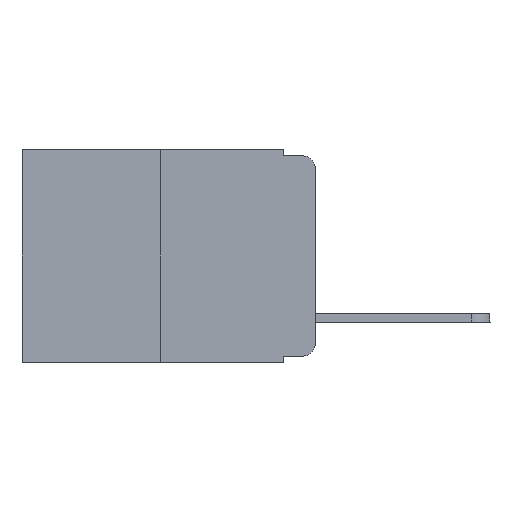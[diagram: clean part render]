
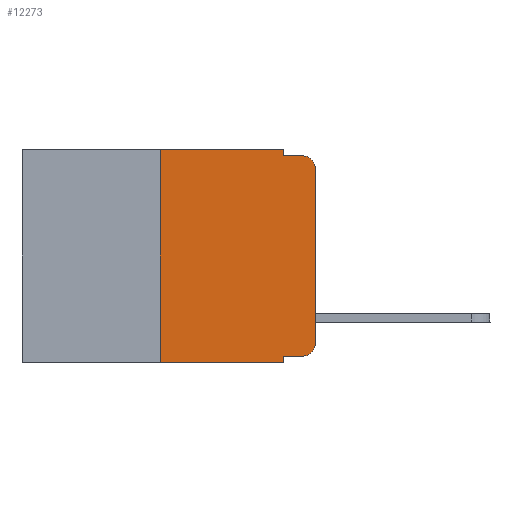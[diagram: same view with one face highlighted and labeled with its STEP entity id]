
A CAD part, left-side view. The second image highlights one B-rep face of the part: STEP entity #12273.
In plain terms, the highlighted planar face has unit normal (-1, 0, 0).
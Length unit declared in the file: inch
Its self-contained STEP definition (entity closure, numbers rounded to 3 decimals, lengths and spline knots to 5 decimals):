
#393 = VERTEX_POINT ( 'NONE', #15303 ) ;
#669 = EDGE_CURVE ( 'NONE', #393, #12281, #3960, .T. ) ;
#1210 = EDGE_CURVE ( 'NONE', #20038, #2780, #21327, .T. ) ;
#1405 = VERTEX_POINT ( 'NONE', #14627 ) ;
#1420 = EDGE_CURVE ( 'NONE', #5129, #18535, #2985, .T. ) ;
#2106 = FACE_OUTER_BOUND ( 'NONE', #10210, .T. ) ;
#2491 = LINE ( 'NONE', #22043, #21456 ) ;
#2536 = EDGE_CURVE ( 'NONE', #1405, #393, #21554, .T. ) ;
#2780 = VERTEX_POINT ( 'NONE', #20606 ) ;
#2985 = LINE ( 'NONE', #23862, #22255 ) ;
#3239 = EDGE_CURVE ( 'NONE', #6194, #11858, #14249, .T. ) ;
#3647 = CARTESIAN_POINT ( 'NONE',  ( 0., 0.02, -0.03 ) ) ;
#3960 = LINE ( 'NONE', #18649, #12678 ) ;
#5054 = ORIENTED_EDGE ( 'NONE', *, *, #14826, .F. ) ;
#5129 = VERTEX_POINT ( 'NONE', #21766 ) ;
#5661 = VECTOR ( 'NONE', #9989, 39.37008 ) ;
#5997 = DIRECTION ( 'NONE',  ( 0., -1., 0. ) ) ;
#6194 = VERTEX_POINT ( 'NONE', #10432 ) ;
#6291 = EDGE_CURVE ( 'NONE', #18881, #18535, #23233, .T. ) ;
#6604 = CARTESIAN_POINT ( 'NONE',  ( 0., 0.25, 0. ) ) ;
#6665 = DIRECTION ( 'NONE',  ( 1., 0., 0. ) ) ;
#6830 = ORIENTED_EDGE ( 'NONE', *, *, #1420, .F. ) ;
#7027 = EDGE_CURVE ( 'NONE', #11858, #20038, #16134, .T. ) ;
#8512 = CARTESIAN_POINT ( 'NONE',  ( 0., 0.051, -0.01 ) ) ;
#8839 = DIRECTION ( 'NONE',  ( 0., 0., -1. ) ) ;
#9484 = ORIENTED_EDGE ( 'NONE', *, *, #10793, .F. ) ;
#9567 = CARTESIAN_POINT ( 'NONE',  ( 0., 0., 0. ) ) ;
#9631 = VECTOR ( 'NONE', #12845, 39.37008 ) ;
#9811 = CARTESIAN_POINT ( 'NONE',  ( 0., 0.051, -0.333 ) ) ;
#9989 = DIRECTION ( 'NONE',  ( 0., -1., 0. ) ) ;
#10210 = EDGE_LOOP ( 'NONE', ( #11267, #16380, #9484, #14131, #15472, #5054, #15921, #6830, #18730, #19516 ) ) ;
#10270 = CARTESIAN_POINT ( 'NONE',  ( 0., 0.473, -0.343 ) ) ;
#10308 = DIRECTION ( 'NONE',  ( -1., 0., 0. ) ) ;
#10432 = CARTESIAN_POINT ( 'NONE',  ( 0., 0.02, -0.333 ) ) ;
#10793 = EDGE_CURVE ( 'NONE', #12281, #2780, #2491, .T. ) ;
#11267 = ORIENTED_EDGE ( 'NONE', *, *, #7027, .T. ) ;
#11858 = VERTEX_POINT ( 'NONE', #16925 ) ;
#12273 = ADVANCED_FACE ( 'NONE', ( #2106 ), #24027, .F. ) ;
#12281 = VERTEX_POINT ( 'NONE', #8512 ) ;
#12386 = DIRECTION ( 'NONE',  ( 0., 0., 1. ) ) ;
#12678 = VECTOR ( 'NONE', #20623, 39.37008 ) ;
#12823 = CARTESIAN_POINT ( 'NONE',  ( 0., 0.051, -0.343 ) ) ;
#12845 = DIRECTION ( 'NONE',  ( 0., -1., 0. ) ) ;
#13366 = CARTESIAN_POINT ( 'NONE',  ( 0., 0., -0.03 ) ) ;
#14131 = ORIENTED_EDGE ( 'NONE', *, *, #669, .F. ) ;
#14249 = CIRCLE ( 'NONE', #18062, 0.02 ) ;
#14353 = DIRECTION ( 'NONE',  ( 0., 0., -1. ) ) ;
#14627 = CARTESIAN_POINT ( 'NONE',  ( 0., 0.25, 0. ) ) ;
#14826 = EDGE_CURVE ( 'NONE', #18881, #1405, #17659, .T. ) ;
#15303 = CARTESIAN_POINT ( 'NONE',  ( 0., 0.051, 0. ) ) ;
#15472 = ORIENTED_EDGE ( 'NONE', *, *, #2536, .F. ) ;
#15921 = ORIENTED_EDGE ( 'NONE', *, *, #6291, .T. ) ;
#16134 = LINE ( 'NONE', #9567, #21299 ) ;
#16195 = CARTESIAN_POINT ( 'NONE',  ( 0., 0.473, 0. ) ) ;
#16380 = ORIENTED_EDGE ( 'NONE', *, *, #1210, .T. ) ;
#16391 = VECTOR ( 'NONE', #5997, 39.37008 ) ;
#16615 = CARTESIAN_POINT ( 'NONE',  ( 0., 0.25, -0.343 ) ) ;
#16925 = CARTESIAN_POINT ( 'NONE',  ( 0., 0., -0.313 ) ) ;
#17659 = LINE ( 'NONE', #6604, #21300 ) ;
#18062 = AXIS2_PLACEMENT_3D ( 'NONE', #19871, #10308, #20043 ) ;
#18535 = VERTEX_POINT ( 'NONE', #12823 ) ;
#18649 = CARTESIAN_POINT ( 'NONE',  ( 0., 0.051, 0. ) ) ;
#18730 = ORIENTED_EDGE ( 'NONE', *, *, #21270, .T. ) ;
#18820 = DIRECTION ( 'NONE',  ( -1., 0., 0. ) ) ;
#18881 = VERTEX_POINT ( 'NONE', #16615 ) ;
#19181 = AXIS2_PLACEMENT_3D ( 'NONE', #16195, #6665, #14353 ) ;
#19462 = DIRECTION ( 'NONE',  ( 0., 0., 1. ) ) ;
#19516 = ORIENTED_EDGE ( 'NONE', *, *, #3239, .T. ) ;
#19520 = CARTESIAN_POINT ( 'NONE',  ( 0., 0.473, 0. ) ) ;
#19871 = CARTESIAN_POINT ( 'NONE',  ( 0., 0.02, -0.313 ) ) ;
#20038 = VERTEX_POINT ( 'NONE', #13366 ) ;
#20043 = DIRECTION ( 'NONE',  ( 0., 0., -1. ) ) ;
#20409 = LINE ( 'NONE', #9811, #5661 ) ;
#20606 = CARTESIAN_POINT ( 'NONE',  ( 0., 0.02, -0.01 ) ) ;
#20623 = DIRECTION ( 'NONE',  ( 0., 0., -1. ) ) ;
#21270 = EDGE_CURVE ( 'NONE', #5129, #6194, #20409, .T. ) ;
#21299 = VECTOR ( 'NONE', #19462, 39.37008 ) ;
#21300 = VECTOR ( 'NONE', #12386, 39.37008 ) ;
#21327 = CIRCLE ( 'NONE', #22311, 0.02 ) ;
#21456 = VECTOR ( 'NONE', #23996, 39.37008 ) ;
#21554 = LINE ( 'NONE', #19520, #16391 ) ;
#21766 = CARTESIAN_POINT ( 'NONE',  ( 0., 0.051, -0.333 ) ) ;
#22043 = CARTESIAN_POINT ( 'NONE',  ( 0., 0.051, -0.01 ) ) ;
#22255 = VECTOR ( 'NONE', #8839, 39.37008 ) ;
#22311 = AXIS2_PLACEMENT_3D ( 'NONE', #3647, #18820, #24872 ) ;
#23233 = LINE ( 'NONE', #10270, #9631 ) ;
#23862 = CARTESIAN_POINT ( 'NONE',  ( 0., 0.051, 0. ) ) ;
#23996 = DIRECTION ( 'NONE',  ( 0., -1., 0. ) ) ;
#24027 = PLANE ( 'NONE',  #19181 ) ;
#24872 = DIRECTION ( 'NONE',  ( 0., 0., -1. ) ) ;
